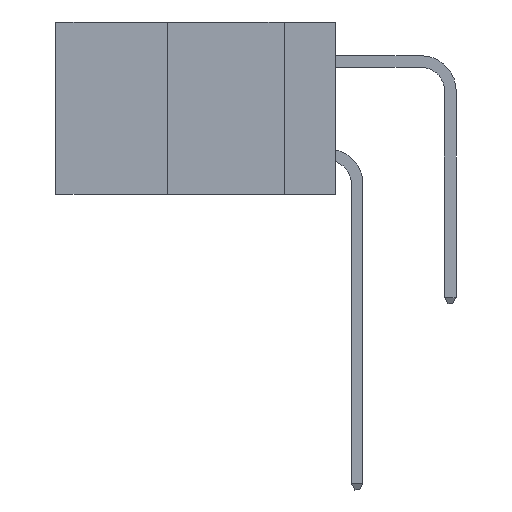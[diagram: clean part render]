
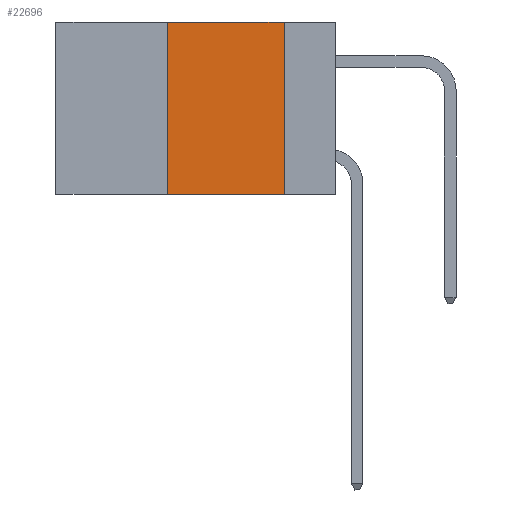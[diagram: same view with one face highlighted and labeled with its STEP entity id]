
A CAD part, left-side view. The second image highlights one B-rep face of the part: STEP entity #22696.
In plain terms, the highlighted planar face has unit normal (-1, 0, 0).
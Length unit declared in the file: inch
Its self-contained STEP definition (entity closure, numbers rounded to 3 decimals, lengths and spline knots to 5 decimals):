
#414 = CARTESIAN_POINT ( 'NONE',  ( 0., 0.6, 0. ) ) ;
#425 = VERTEX_POINT ( 'NONE', #28371 ) ;
#2318 = DIRECTION ( 'NONE',  ( 0., 0., -1. ) ) ;
#2842 = LINE ( 'NONE', #4944, #27838 ) ;
#4266 = ORIENTED_EDGE ( 'NONE', *, *, #25777, .T. ) ;
#4944 = CARTESIAN_POINT ( 'NONE',  ( 0., 0.11, 0. ) ) ;
#6545 = CARTESIAN_POINT ( 'NONE',  ( 0., 0.11, 0. ) ) ;
#7209 = EDGE_CURVE ( 'NONE', #13004, #425, #2842, .T. ) ;
#7721 = EDGE_CURVE ( 'NONE', #20233, #9723, #25451, .T. ) ;
#7811 = DIRECTION ( 'NONE',  ( 0., -1., 0. ) ) ;
#8170 = ORIENTED_EDGE ( 'NONE', *, *, #31361, .F. ) ;
#9723 = VERTEX_POINT ( 'NONE', #30585 ) ;
#9957 = AXIS2_PLACEMENT_3D ( 'NONE', #414, #17736, #30661 ) ;
#10375 = EDGE_LOOP ( 'NONE', ( #13597, #8170, #26645, #4266 ) ) ;
#10396 = LINE ( 'NONE', #21208, #30275 ) ;
#13004 = VERTEX_POINT ( 'NONE', #6545 ) ;
#13280 = DIRECTION ( 'NONE',  ( 0., -1., 0. ) ) ;
#13597 = ORIENTED_EDGE ( 'NONE', *, *, #7209, .F. ) ;
#15254 = CARTESIAN_POINT ( 'NONE',  ( 0., 0.6, 0. ) ) ;
#15849 = LINE ( 'NONE', #15254, #30905 ) ;
#16914 = DIRECTION ( 'NONE',  ( 0., 0., 1. ) ) ;
#17254 = CARTESIAN_POINT ( 'NONE',  ( 0., 0.36, 0. ) ) ;
#17736 = DIRECTION ( 'NONE',  ( 1., 0., 0. ) ) ;
#20233 = VERTEX_POINT ( 'NONE', #31555 ) ;
#21208 = CARTESIAN_POINT ( 'NONE',  ( 0., 0.6, -0.37 ) ) ;
#22696 = ADVANCED_FACE ( 'NONE', ( #29282 ), #27846, .F. ) ;
#25451 = LINE ( 'NONE', #17254, #27812 ) ;
#25777 = EDGE_CURVE ( 'NONE', #20233, #425, #10396, .T. ) ;
#26645 = ORIENTED_EDGE ( 'NONE', *, *, #7721, .F. ) ;
#27812 = VECTOR ( 'NONE', #16914, 39.37008 ) ;
#27838 = VECTOR ( 'NONE', #2318, 39.37008 ) ;
#27846 = PLANE ( 'NONE',  #9957 ) ;
#28371 = CARTESIAN_POINT ( 'NONE',  ( 0., 0.11, -0.37 ) ) ;
#29282 = FACE_OUTER_BOUND ( 'NONE', #10375, .T. ) ;
#30275 = VECTOR ( 'NONE', #13280, 39.37008 ) ;
#30585 = CARTESIAN_POINT ( 'NONE',  ( 0., 0.36, 0. ) ) ;
#30661 = DIRECTION ( 'NONE',  ( 0., 0., -1. ) ) ;
#30905 = VECTOR ( 'NONE', #7811, 39.37008 ) ;
#31361 = EDGE_CURVE ( 'NONE', #9723, #13004, #15849, .T. ) ;
#31555 = CARTESIAN_POINT ( 'NONE',  ( 0., 0.36, -0.37 ) ) ;
